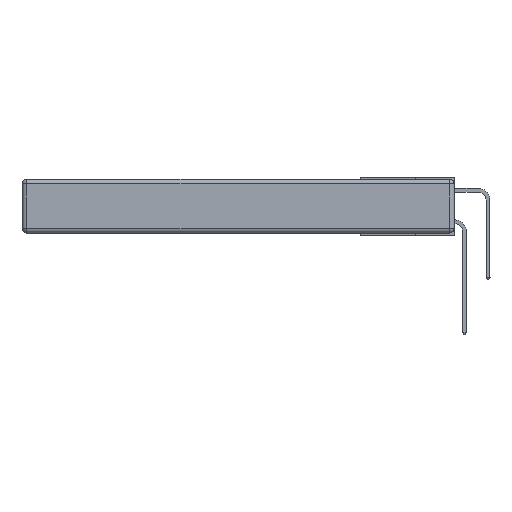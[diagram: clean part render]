
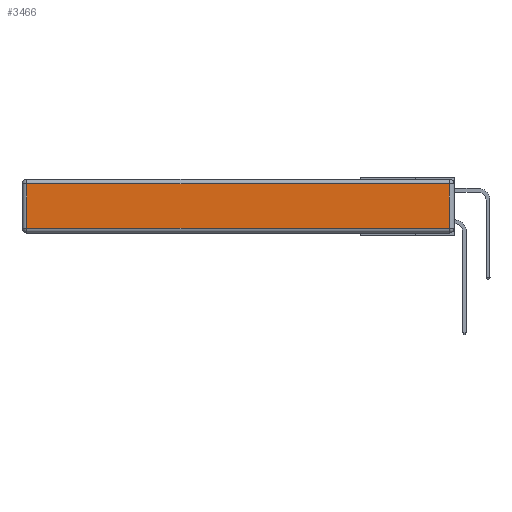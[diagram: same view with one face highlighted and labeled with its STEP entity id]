
A CAD part, left-side view. The second image highlights one B-rep face of the part: STEP entity #3466.
In plain terms, the highlighted planar face has unit normal (-1, 0, 0).
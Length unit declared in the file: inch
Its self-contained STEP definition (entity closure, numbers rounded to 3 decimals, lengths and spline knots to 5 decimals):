
#233 = VECTOR ( 'NONE', #846, 39.37008 ) ;
#373 = DIRECTION ( 'NONE',  ( 0., -1., 0. ) ) ;
#467 = CARTESIAN_POINT ( 'NONE',  ( 0., 0., -0.313 ) ) ;
#846 = DIRECTION ( 'NONE',  ( 0., 0., -1. ) ) ;
#1344 = EDGE_CURVE ( 'NONE', #4537, #4280, #20232, .T. ) ;
#3466 = ADVANCED_FACE ( 'NONE', ( #16605 ), #22648, .T. ) ;
#4280 = VERTEX_POINT ( 'NONE', #12768 ) ;
#4389 = EDGE_CURVE ( 'NONE', #6228, #4537, #11599, .T. ) ;
#4537 = VERTEX_POINT ( 'NONE', #16795 ) ;
#4954 = CARTESIAN_POINT ( 'NONE',  ( 0., 0.03, -0.313 ) ) ;
#5134 = ORIENTED_EDGE ( 'NONE', *, *, #1344, .T. ) ;
#6228 = VERTEX_POINT ( 'NONE', #4954 ) ;
#6322 = VECTOR ( 'NONE', #6909, 39.37008 ) ;
#6909 = DIRECTION ( 'NONE',  ( 0., 0., 1. ) ) ;
#7963 = ORIENTED_EDGE ( 'NONE', *, *, #20292, .T. ) ;
#8303 = CARTESIAN_POINT ( 'NONE',  ( 0., 2.72, -0.313 ) ) ;
#8574 = DIRECTION ( 'NONE',  ( 0., 1., 0. ) ) ;
#8651 = VERTEX_POINT ( 'NONE', #8303 ) ;
#8726 = CARTESIAN_POINT ( 'NONE',  ( 0., 0.03, -0.343 ) ) ;
#9342 = DIRECTION ( 'NONE',  ( 0., 0., 1. ) ) ;
#9932 = LINE ( 'NONE', #14100, #233 ) ;
#10472 = EDGE_CURVE ( 'NONE', #4280, #8651, #9932, .T. ) ;
#11146 = CARTESIAN_POINT ( 'NONE',  ( 0., 0., -0.343 ) ) ;
#11599 = LINE ( 'NONE', #8726, #6322 ) ;
#12318 = VECTOR ( 'NONE', #8574, 39.37008 ) ;
#12328 = ORIENTED_EDGE ( 'NONE', *, *, #10472, .T. ) ;
#12768 = CARTESIAN_POINT ( 'NONE',  ( 0., 2.72, -0.03 ) ) ;
#13004 = DIRECTION ( 'NONE',  ( -1., 0., 0. ) ) ;
#13954 = EDGE_LOOP ( 'NONE', ( #7963, #24038, #5134, #12328 ) ) ;
#14100 = CARTESIAN_POINT ( 'NONE',  ( 0., 2.72, -0.343 ) ) ;
#14473 = CARTESIAN_POINT ( 'NONE',  ( 0., 2.75, -0.03 ) ) ;
#15502 = AXIS2_PLACEMENT_3D ( 'NONE', #11146, #13004, #9342 ) ;
#15981 = VECTOR ( 'NONE', #373, 39.37008 ) ;
#16605 = FACE_OUTER_BOUND ( 'NONE', #13954, .T. ) ;
#16795 = CARTESIAN_POINT ( 'NONE',  ( 0., 0.03, -0.03 ) ) ;
#18931 = LINE ( 'NONE', #467, #15981 ) ;
#20232 = LINE ( 'NONE', #14473, #12318 ) ;
#20292 = EDGE_CURVE ( 'NONE', #8651, #6228, #18931, .T. ) ;
#22648 = PLANE ( 'NONE',  #15502 ) ;
#24038 = ORIENTED_EDGE ( 'NONE', *, *, #4389, .T. ) ;
